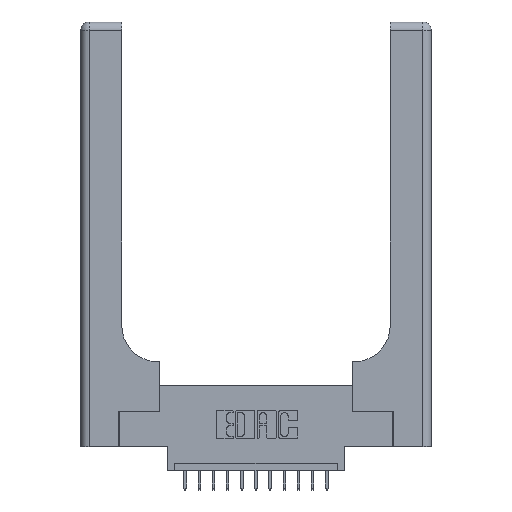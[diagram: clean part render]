
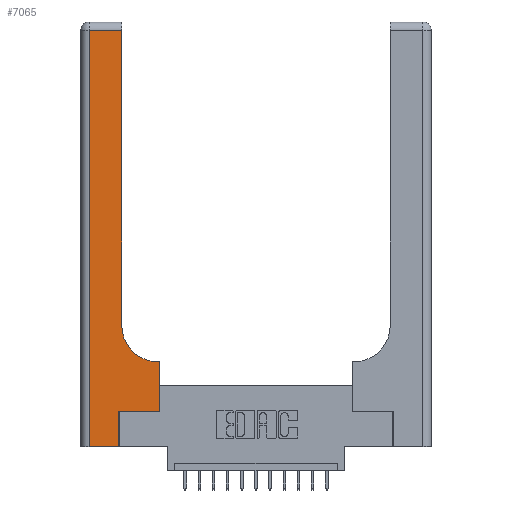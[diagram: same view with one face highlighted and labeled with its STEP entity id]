
A CAD part, top view. The second image highlights one B-rep face of the part: STEP entity #7065.
In plain terms, the highlighted planar face has unit normal (0, 0, 1).
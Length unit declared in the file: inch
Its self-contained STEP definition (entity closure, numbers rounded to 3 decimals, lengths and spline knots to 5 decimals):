
#223 = CARTESIAN_POINT ( 'NONE',  ( 0.269, 0.25, 0.37 ) ) ;
#533 = CARTESIAN_POINT ( 'NONE',  ( 0.269, 0., 0.37 ) ) ;
#715 = LINE ( 'NONE', #533, #11135 ) ;
#945 = VERTEX_POINT ( 'NONE', #2132 ) ;
#1141 = VECTOR ( 'NONE', #17425, 39.37008 ) ;
#1350 = LINE ( 'NONE', #5682, #14843 ) ;
#1378 = DIRECTION ( 'NONE',  ( 0., 0., -1. ) ) ;
#1756 = VECTOR ( 'NONE', #15158, 39.37008 ) ;
#2012 = ORIENTED_EDGE ( 'NONE', *, *, #16986, .T. ) ;
#2132 = CARTESIAN_POINT ( 'NONE',  ( 0.5415, 0.6, 0.37 ) ) ;
#2134 = DIRECTION ( 'NONE',  ( 0., 1., 0. ) ) ;
#2361 = AXIS2_PLACEMENT_3D ( 'NONE', #15623, #6119, #10188 ) ;
#2662 = ORIENTED_EDGE ( 'NONE', *, *, #3020, .T. ) ;
#2747 = CARTESIAN_POINT ( 'NONE',  ( 0.5415, 0.85, 0.37 ) ) ;
#3020 = EDGE_CURVE ( 'NONE', #17752, #12189, #15631, .T. ) ;
#3024 = CARTESIAN_POINT ( 'NONE',  ( 0.06, 3., 0.37 ) ) ;
#3126 = ORIENTED_EDGE ( 'NONE', *, *, #14945, .T. ) ;
#3226 = CARTESIAN_POINT ( 'NONE',  ( 0.2915, 0.6, 0.37 ) ) ;
#3252 = PLANE ( 'NONE',  #2361 ) ;
#3262 = CARTESIAN_POINT ( 'NONE',  ( 0.5585, 0.25, 0.37 ) ) ;
#3393 = EDGE_CURVE ( 'NONE', #6069, #17752, #10988, .T. ) ;
#3752 = ORIENTED_EDGE ( 'NONE', *, *, #6622, .T. ) ;
#4276 = CARTESIAN_POINT ( 'NONE',  ( 0.5585, 0.25, 0.37 ) ) ;
#4825 = CARTESIAN_POINT ( 'NONE',  ( 0.5585, 0.6, 0.37 ) ) ;
#5222 = VECTOR ( 'NONE', #2134, 39.37008 ) ;
#5345 = CARTESIAN_POINT ( 'NONE',  ( 0.06, 2.94, 0.37 ) ) ;
#5543 = LINE ( 'NONE', #3024, #11996 ) ;
#5682 = CARTESIAN_POINT ( 'NONE',  ( 0., 2.94, 0.37 ) ) ;
#5943 = EDGE_CURVE ( 'NONE', #15659, #10693, #14425, .T. ) ;
#6047 = VERTEX_POINT ( 'NONE', #16484 ) ;
#6069 = VERTEX_POINT ( 'NONE', #17751 ) ;
#6119 = DIRECTION ( 'NONE',  ( 0., 0., -1. ) ) ;
#6209 = FACE_OUTER_BOUND ( 'NONE', #17868, .T. ) ;
#6622 = EDGE_CURVE ( 'NONE', #945, #15659, #10418, .T. ) ;
#6816 = VERTEX_POINT ( 'NONE', #5345 ) ;
#6888 = DIRECTION ( 'NONE',  ( 1., 0., 0. ) ) ;
#7065 = ADVANCED_FACE ( 'NONE', ( #6209 ), #3252, .F. ) ;
#7856 = ORIENTED_EDGE ( 'NONE', *, *, #10097, .T. ) ;
#7932 = DIRECTION ( 'NONE',  ( 1., 0., 0. ) ) ;
#8465 = ORIENTED_EDGE ( 'NONE', *, *, #12742, .T. ) ;
#8883 = ORIENTED_EDGE ( 'NONE', *, *, #5943, .T. ) ;
#9533 = AXIS2_PLACEMENT_3D ( 'NONE', #2747, #1378, #6888 ) ;
#9903 = LINE ( 'NONE', #3226, #13203 ) ;
#10097 = EDGE_CURVE ( 'NONE', #10693, #6816, #1350, .T. ) ;
#10188 = DIRECTION ( 'NONE',  ( -1., 0., 0. ) ) ;
#10410 = CARTESIAN_POINT ( 'NONE',  ( 0.2915, 2.94, 0.37 ) ) ;
#10418 = CIRCLE ( 'NONE', #9533, 0.25 ) ;
#10693 = VERTEX_POINT ( 'NONE', #10410 ) ;
#10988 = LINE ( 'NONE', #223, #1756 ) ;
#11057 = DIRECTION ( 'NONE',  ( 0., -1., 0. ) ) ;
#11135 = VECTOR ( 'NONE', #14279, 39.37008 ) ;
#11996 = VECTOR ( 'NONE', #11057, 39.37008 ) ;
#12099 = CARTESIAN_POINT ( 'NONE',  ( 0., 0., 0.37 ) ) ;
#12189 = VERTEX_POINT ( 'NONE', #4825 ) ;
#12393 = VERTEX_POINT ( 'NONE', #14456 ) ;
#12742 = EDGE_CURVE ( 'NONE', #6816, #12393, #5543, .T. ) ;
#13022 = ORIENTED_EDGE ( 'NONE', *, *, #13263, .T. ) ;
#13203 = VECTOR ( 'NONE', #14161, 39.37008 ) ;
#13263 = EDGE_CURVE ( 'NONE', #6047, #6069, #715, .T. ) ;
#13745 = DIRECTION ( 'NONE',  ( -1., 0., 0. ) ) ;
#13802 = ORIENTED_EDGE ( 'NONE', *, *, #3393, .T. ) ;
#14058 = VECTOR ( 'NONE', #7932, 39.37008 ) ;
#14161 = DIRECTION ( 'NONE',  ( -1., 0., 0. ) ) ;
#14279 = DIRECTION ( 'NONE',  ( 0., 1., 0. ) ) ;
#14425 = LINE ( 'NONE', #17127, #5222 ) ;
#14456 = CARTESIAN_POINT ( 'NONE',  ( 0.06, 0., 0.37 ) ) ;
#14843 = VECTOR ( 'NONE', #13745, 39.37008 ) ;
#14945 = EDGE_CURVE ( 'NONE', #12393, #6047, #17669, .T. ) ;
#15158 = DIRECTION ( 'NONE',  ( 1., 0., 0. ) ) ;
#15623 = CARTESIAN_POINT ( 'NONE',  ( 0., 3., 0.37 ) ) ;
#15631 = LINE ( 'NONE', #3262, #1141 ) ;
#15659 = VERTEX_POINT ( 'NONE', #17008 ) ;
#16484 = CARTESIAN_POINT ( 'NONE',  ( 0.269, 0., 0.37 ) ) ;
#16986 = EDGE_CURVE ( 'NONE', #12189, #945, #9903, .T. ) ;
#17008 = CARTESIAN_POINT ( 'NONE',  ( 0.2915, 0.85, 0.37 ) ) ;
#17127 = CARTESIAN_POINT ( 'NONE',  ( 0.2915, 3., 0.37 ) ) ;
#17425 = DIRECTION ( 'NONE',  ( 0., 1., 0. ) ) ;
#17669 = LINE ( 'NONE', #12099, #14058 ) ;
#17751 = CARTESIAN_POINT ( 'NONE',  ( 0.269, 0.25, 0.37 ) ) ;
#17752 = VERTEX_POINT ( 'NONE', #4276 ) ;
#17868 = EDGE_LOOP ( 'NONE', ( #8883, #7856, #8465, #3126, #13022, #13802, #2662, #2012, #3752 ) ) ;
